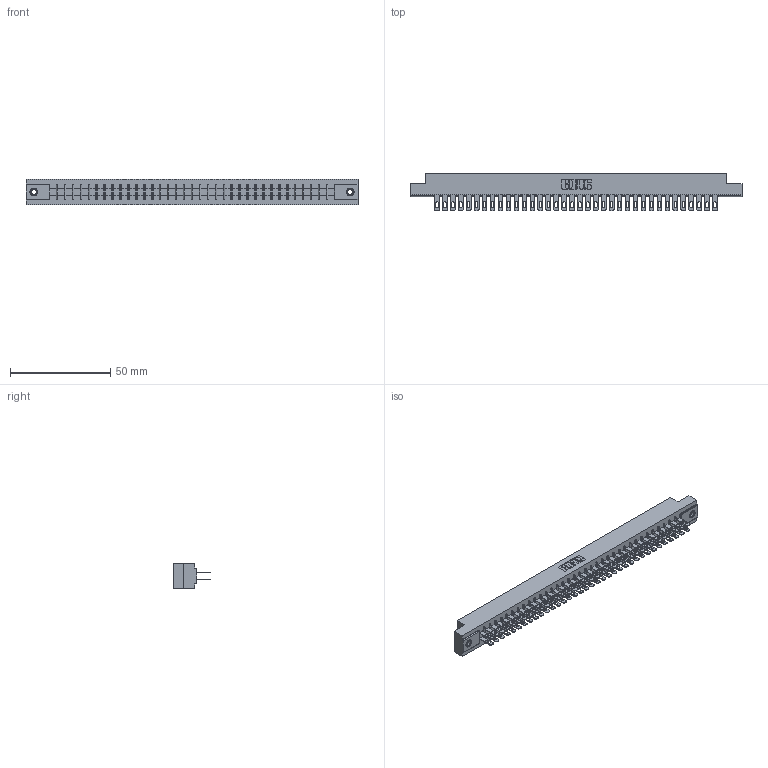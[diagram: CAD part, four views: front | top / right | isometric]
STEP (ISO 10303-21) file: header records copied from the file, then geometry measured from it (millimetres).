
FILE_DESCRIPTION (( 'STEP AP203' ), '1' );
FILE_NAME ('355-072-500-207.STEP', '2019-09-12T17:51:00', ( '' ), ( '' ), 'SwSTEP 2.0', 'SolidWorks 2016', '' );
FILE_SCHEMA (( 'CONFIG_CONTROL_DESIGN' ));
Length unit declared in the file: inch
Products named in the file (4): 355-072-500-207; 305 Part_.156 Dia; 345-250-001_345-250-005-103; 305-290-001_500
Assembly tree (75 placements, depth 2):
  355-072-500-207
    305 Part_.156 Dia
    305-290-001_500  x72
    345-250-001_345-250-005-103  x2
Bounding box: 165.66 x 18.85 x 12.7 mm (x, y, z)
Volume: 17449.5 mm3; surface area: 23517.1 mm2
Topology: 75 solids, 75 shells, 3776 faces, 10784 edges, 6988 vertices
Faces by surface type: plane 2116, cylinder 1500, sphere 144, cone 12, torus 4
Entity records: 40916 total; most frequent: CARTESIAN_POINT 6753, ORIENTED_EDGE 6696, DIRECTION 6550, EDGE_CURVE 3348, LINE 2696, VECTOR 2696, VERTEX_POINT 2130, AXIS2_PLACEMENT_3D 1927
